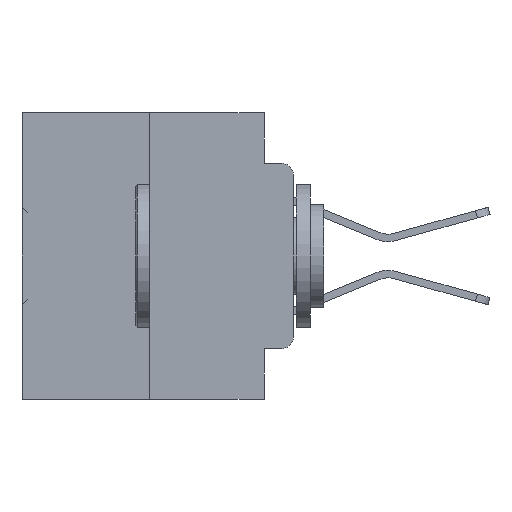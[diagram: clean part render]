
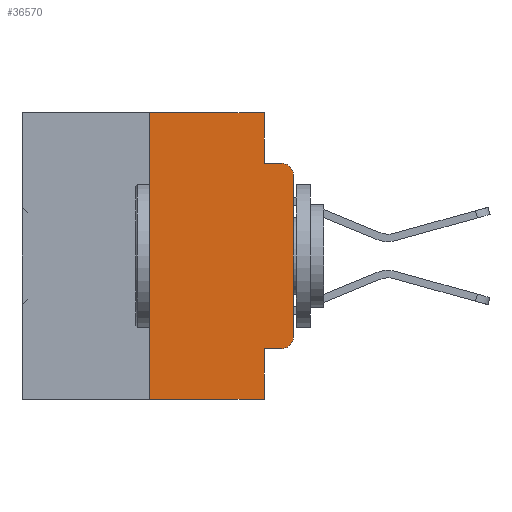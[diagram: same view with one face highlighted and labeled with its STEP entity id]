
A CAD part, left-side view. The second image highlights one B-rep face of the part: STEP entity #36570.
In plain terms, the highlighted planar face has unit normal (-1, 0, 0).
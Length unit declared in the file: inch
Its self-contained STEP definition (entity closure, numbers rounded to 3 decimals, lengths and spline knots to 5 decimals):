
#79 = LINE ( 'NONE', #17694, #1187 ) ;
#1088 = DIRECTION ( 'NONE',  ( 0., 0., -1. ) ) ;
#1187 = VECTOR ( 'NONE', #23616, 39.37008 ) ;
#1457 = EDGE_CURVE ( 'NONE', #29875, #23667, #20433, .T. ) ;
#2227 = ORIENTED_EDGE ( 'NONE', *, *, #22320, .T. ) ;
#2366 = DIRECTION ( 'NONE',  ( 0., -1., 0. ) ) ;
#2691 = CARTESIAN_POINT ( 'NONE',  ( 0., 0.051, -0.5 ) ) ;
#3398 = DIRECTION ( 'NONE',  ( 0., 0., -1. ) ) ;
#3596 = CARTESIAN_POINT ( 'NONE',  ( 0., 0.051, 0. ) ) ;
#3734 = VERTEX_POINT ( 'NONE', #19408 ) ;
#3961 = CARTESIAN_POINT ( 'NONE',  ( 0., 0.473, -0.5 ) ) ;
#4331 = LINE ( 'NONE', #3961, #32791 ) ;
#5239 = EDGE_CURVE ( 'NONE', #37627, #16105, #79, .T. ) ;
#5293 = ORIENTED_EDGE ( 'NONE', *, *, #11247, .T. ) ;
#5544 = CARTESIAN_POINT ( 'NONE',  ( 0., 0.02, -0.4115 ) ) ;
#7491 = CARTESIAN_POINT ( 'NONE',  ( 0., 0.02, -0.1085 ) ) ;
#7879 = CARTESIAN_POINT ( 'NONE',  ( 0., 0., -0.1085 ) ) ;
#8335 = DIRECTION ( 'NONE',  ( 0., -1., 0. ) ) ;
#8503 = EDGE_CURVE ( 'NONE', #3734, #33194, #27251, .T. ) ;
#8639 = EDGE_CURVE ( 'NONE', #16105, #37471, #16448, .T. ) ;
#8827 = EDGE_CURVE ( 'NONE', #14259, #26714, #25556, .T. ) ;
#9150 = CARTESIAN_POINT ( 'NONE',  ( 0., 0.051, 0. ) ) ;
#10546 = CARTESIAN_POINT ( 'NONE',  ( 0., 0., -0.3915 ) ) ;
#10741 = EDGE_CURVE ( 'NONE', #26714, #37627, #37163, .T. ) ;
#11247 = EDGE_CURVE ( 'NONE', #23667, #37471, #18460, .T. ) ;
#11667 = EDGE_CURVE ( 'NONE', #3734, #22840, #34896, .T. ) ;
#11910 = CIRCLE ( 'NONE', #29601, 0.02 ) ;
#12941 = FACE_OUTER_BOUND ( 'NONE', #23476, .T. ) ;
#12970 = AXIS2_PLACEMENT_3D ( 'NONE', #7491, #28517, #22810 ) ;
#13137 = DIRECTION ( 'NONE',  ( 0., 0., -1. ) ) ;
#13193 = CARTESIAN_POINT ( 'NONE',  ( 0., 0.25, -0.5 ) ) ;
#13312 = CARTESIAN_POINT ( 'NONE',  ( 0., 0.473, 0. ) ) ;
#14259 = VERTEX_POINT ( 'NONE', #13193 ) ;
#14587 = ORIENTED_EDGE ( 'NONE', *, *, #8639, .F. ) ;
#14907 = CARTESIAN_POINT ( 'NONE',  ( 0., 0.02, -0.3915 ) ) ;
#15846 = CARTESIAN_POINT ( 'NONE',  ( 0., 0.051, -0.0885 ) ) ;
#15966 = ORIENTED_EDGE ( 'NONE', *, *, #11667, .T. ) ;
#16105 = VERTEX_POINT ( 'NONE', #20944 ) ;
#16448 = LINE ( 'NONE', #15846, #37710 ) ;
#17694 = CARTESIAN_POINT ( 'NONE',  ( 0., 0.051, 0. ) ) ;
#18460 = CIRCLE ( 'NONE', #12970, 0.02 ) ;
#19056 = PLANE ( 'NONE',  #23299 ) ;
#19394 = EDGE_CURVE ( 'NONE', #22840, #29875, #11910, .T. ) ;
#19408 = CARTESIAN_POINT ( 'NONE',  ( 0., 0.051, -0.4115 ) ) ;
#20433 = LINE ( 'NONE', #21181, #26852 ) ;
#20944 = CARTESIAN_POINT ( 'NONE',  ( 0., 0.051, -0.0885 ) ) ;
#20999 = CARTESIAN_POINT ( 'NONE',  ( 0., 0.25, 0. ) ) ;
#21181 = CARTESIAN_POINT ( 'NONE',  ( 0., 0., 0. ) ) ;
#21892 = VECTOR ( 'NONE', #30107, 39.37008 ) ;
#22132 = VECTOR ( 'NONE', #8335, 39.37008 ) ;
#22320 = EDGE_CURVE ( 'NONE', #14259, #33194, #4331, .T. ) ;
#22810 = DIRECTION ( 'NONE',  ( 0., 0., -1. ) ) ;
#22840 = VERTEX_POINT ( 'NONE', #5544 ) ;
#23018 = ORIENTED_EDGE ( 'NONE', *, *, #8827, .F. ) ;
#23299 = AXIS2_PLACEMENT_3D ( 'NONE', #13312, #27999, #13137 ) ;
#23476 = EDGE_LOOP ( 'NONE', ( #36437, #5293, #14587, #33078, #29299, #23018, #2227, #27917, #15966, #30199 ) ) ;
#23616 = DIRECTION ( 'NONE',  ( 0., 0., -1. ) ) ;
#23667 = VERTEX_POINT ( 'NONE', #7879 ) ;
#23674 = DIRECTION ( 'NONE',  ( -1., 0., 0. ) ) ;
#25318 = CARTESIAN_POINT ( 'NONE',  ( 0., 0.473, 0. ) ) ;
#25556 = LINE ( 'NONE', #20999, #21892 ) ;
#26106 = CARTESIAN_POINT ( 'NONE',  ( 0., 0.051, -0.4115 ) ) ;
#26714 = VERTEX_POINT ( 'NONE', #37000 ) ;
#26852 = VECTOR ( 'NONE', #35674, 39.37008 ) ;
#27251 = LINE ( 'NONE', #9150, #29115 ) ;
#27440 = DIRECTION ( 'NONE',  ( 0., -1., 0. ) ) ;
#27917 = ORIENTED_EDGE ( 'NONE', *, *, #8503, .F. ) ;
#27999 = DIRECTION ( 'NONE',  ( 1., 0., 0. ) ) ;
#28517 = DIRECTION ( 'NONE',  ( -1., 0., 0. ) ) ;
#29115 = VECTOR ( 'NONE', #1088, 39.37008 ) ;
#29299 = ORIENTED_EDGE ( 'NONE', *, *, #10741, .F. ) ;
#29402 = VECTOR ( 'NONE', #2366, 39.37008 ) ;
#29601 = AXIS2_PLACEMENT_3D ( 'NONE', #14907, #23674, #3398 ) ;
#29875 = VERTEX_POINT ( 'NONE', #10546 ) ;
#30107 = DIRECTION ( 'NONE',  ( 0., 0., 1. ) ) ;
#30199 = ORIENTED_EDGE ( 'NONE', *, *, #19394, .T. ) ;
#32112 = CARTESIAN_POINT ( 'NONE',  ( 0., 0.02, -0.0885 ) ) ;
#32791 = VECTOR ( 'NONE', #33217, 39.37008 ) ;
#33078 = ORIENTED_EDGE ( 'NONE', *, *, #5239, .F. ) ;
#33194 = VERTEX_POINT ( 'NONE', #2691 ) ;
#33217 = DIRECTION ( 'NONE',  ( 0., -1., 0. ) ) ;
#34896 = LINE ( 'NONE', #26106, #22132 ) ;
#35674 = DIRECTION ( 'NONE',  ( 0., 0., 1. ) ) ;
#36437 = ORIENTED_EDGE ( 'NONE', *, *, #1457, .T. ) ;
#36570 = ADVANCED_FACE ( 'NONE', ( #12941 ), #19056, .F. ) ;
#37000 = CARTESIAN_POINT ( 'NONE',  ( 0., 0.25, 0. ) ) ;
#37163 = LINE ( 'NONE', #25318, #29402 ) ;
#37471 = VERTEX_POINT ( 'NONE', #32112 ) ;
#37627 = VERTEX_POINT ( 'NONE', #3596 ) ;
#37710 = VECTOR ( 'NONE', #27440, 39.37008 ) ;
